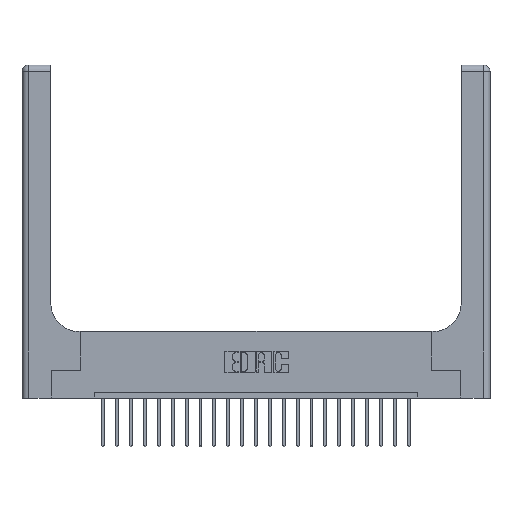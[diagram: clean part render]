
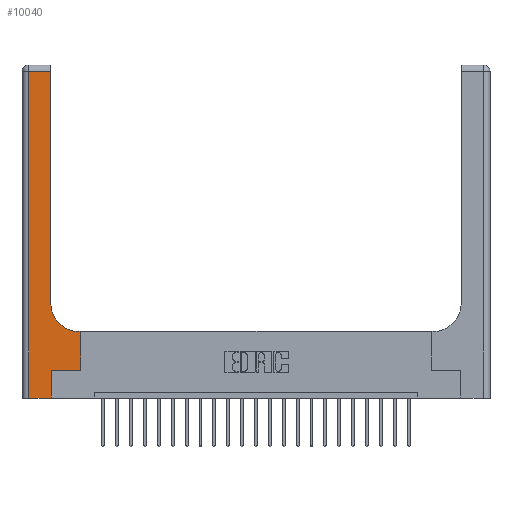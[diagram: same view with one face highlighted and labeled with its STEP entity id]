
A CAD part, top view. The second image highlights one B-rep face of the part: STEP entity #10040.
In plain terms, the highlighted planar face has unit normal (0, 0, 1).
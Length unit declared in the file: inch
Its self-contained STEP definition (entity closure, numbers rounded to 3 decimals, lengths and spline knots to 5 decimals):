
#422 = EDGE_CURVE ( 'NONE', #13824, #6355, #600, .T. ) ;
#600 = LINE ( 'NONE', #7864, #15520 ) ;
#1306 = VECTOR ( 'NONE', #3879, 39.37008 ) ;
#1350 = ORIENTED_EDGE ( 'NONE', *, *, #422, .T. ) ;
#1509 = DIRECTION ( 'NONE',  ( -1., 0., 0. ) ) ;
#1542 = ORIENTED_EDGE ( 'NONE', *, *, #16143, .T. ) ;
#1742 = CARTESIAN_POINT ( 'NONE',  ( 0.528, 0.25, 0.37 ) ) ;
#1911 = ORIENTED_EDGE ( 'NONE', *, *, #18647, .T. ) ;
#3413 = CARTESIAN_POINT ( 'NONE',  ( 0.51, 0.6, 0.37 ) ) ;
#3441 = DIRECTION ( 'NONE',  ( 0., 1., 0. ) ) ;
#3488 = AXIS2_PLACEMENT_3D ( 'NONE', #11070, #20191, #18031 ) ;
#3821 = VECTOR ( 'NONE', #7078, 39.37008 ) ;
#3879 = DIRECTION ( 'NONE',  ( 0., 1., 0. ) ) ;
#4105 = CARTESIAN_POINT ( 'NONE',  ( 0.06, 0., 0.37 ) ) ;
#4559 = LINE ( 'NONE', #14775, #11260 ) ;
#4609 = LINE ( 'NONE', #16997, #16040 ) ;
#4688 = CARTESIAN_POINT ( 'NONE',  ( 0.528, 0.25, 0.37 ) ) ;
#5566 = PLANE ( 'NONE',  #7668 ) ;
#5663 = VECTOR ( 'NONE', #21361, 39.37008 ) ;
#6355 = VERTEX_POINT ( 'NONE', #4105 ) ;
#7029 = VERTEX_POINT ( 'NONE', #4688 ) ;
#7078 = DIRECTION ( 'NONE',  ( -1., 0., 0. ) ) ;
#7214 = EDGE_CURVE ( 'NONE', #20038, #16830, #14089, .T. ) ;
#7511 = CARTESIAN_POINT ( 'NONE',  ( 0.26, 0.85, 0.37 ) ) ;
#7668 = AXIS2_PLACEMENT_3D ( 'NONE', #15899, #13770, #1509 ) ;
#7864 = CARTESIAN_POINT ( 'NONE',  ( 0.06, 3., 0.37 ) ) ;
#8215 = EDGE_CURVE ( 'NONE', #7029, #13641, #22311, .T. ) ;
#8663 = VERTEX_POINT ( 'NONE', #3413 ) ;
#8960 = CARTESIAN_POINT ( 'NONE',  ( 0.265, 0.25, 0.37 ) ) ;
#9094 = LINE ( 'NONE', #17748, #21242 ) ;
#9888 = DIRECTION ( 'NONE',  ( -1., 0., 0. ) ) ;
#10040 = ADVANCED_FACE ( 'NONE', ( #21147 ), #5566, .F. ) ;
#10306 = ORIENTED_EDGE ( 'NONE', *, *, #10682, .T. ) ;
#10348 = CARTESIAN_POINT ( 'NONE',  ( 0.06, 2.94, 0.37 ) ) ;
#10359 = CARTESIAN_POINT ( 'NONE',  ( 0.26, 0.6, 0.37 ) ) ;
#10680 = CARTESIAN_POINT ( 'NONE',  ( 0.265, 0., 0.37 ) ) ;
#10682 = EDGE_CURVE ( 'NONE', #6355, #20038, #4609, .T. ) ;
#10888 = ORIENTED_EDGE ( 'NONE', *, *, #16831, .T. ) ;
#11070 = CARTESIAN_POINT ( 'NONE',  ( 0.51, 0.85, 0.37 ) ) ;
#11137 = EDGE_CURVE ( 'NONE', #14824, #13824, #4559, .T. ) ;
#11260 = VECTOR ( 'NONE', #9888, 39.37008 ) ;
#12115 = CARTESIAN_POINT ( 'NONE',  ( 0.528, 0.6, 0.37 ) ) ;
#12662 = ORIENTED_EDGE ( 'NONE', *, *, #11137, .T. ) ;
#12752 = DIRECTION ( 'NONE',  ( 0., -1., 0. ) ) ;
#13272 = CIRCLE ( 'NONE', #3488, 0.25 ) ;
#13641 = VERTEX_POINT ( 'NONE', #12115 ) ;
#13657 = LINE ( 'NONE', #10359, #3821 ) ;
#13687 = DIRECTION ( 'NONE',  ( 1., 0., 0. ) ) ;
#13770 = DIRECTION ( 'NONE',  ( 0., 0., -1. ) ) ;
#13824 = VERTEX_POINT ( 'NONE', #10348 ) ;
#13974 = VERTEX_POINT ( 'NONE', #7511 ) ;
#14089 = LINE ( 'NONE', #10680, #1306 ) ;
#14172 = LINE ( 'NONE', #15785, #5663 ) ;
#14683 = EDGE_LOOP ( 'NONE', ( #10888, #12662, #1350, #10306, #16465, #15661, #21890, #1542, #1911 ) ) ;
#14775 = CARTESIAN_POINT ( 'NONE',  ( 0., 2.94, 0.37 ) ) ;
#14824 = VERTEX_POINT ( 'NONE', #21982 ) ;
#15520 = VECTOR ( 'NONE', #12752, 39.37008 ) ;
#15661 = ORIENTED_EDGE ( 'NONE', *, *, #17598, .T. ) ;
#15785 = CARTESIAN_POINT ( 'NONE',  ( 0.26, 3., 0.37 ) ) ;
#15899 = CARTESIAN_POINT ( 'NONE',  ( 0., 3., 0.37 ) ) ;
#16040 = VECTOR ( 'NONE', #13687, 39.37008 ) ;
#16143 = EDGE_CURVE ( 'NONE', #13641, #8663, #13657, .T. ) ;
#16465 = ORIENTED_EDGE ( 'NONE', *, *, #7214, .T. ) ;
#16830 = VERTEX_POINT ( 'NONE', #8960 ) ;
#16831 = EDGE_CURVE ( 'NONE', #13974, #14824, #14172, .T. ) ;
#16997 = CARTESIAN_POINT ( 'NONE',  ( 0., 0., 0.37 ) ) ;
#17598 = EDGE_CURVE ( 'NONE', #16830, #7029, #9094, .T. ) ;
#17748 = CARTESIAN_POINT ( 'NONE',  ( 0.265, 0.25, 0.37 ) ) ;
#17934 = VECTOR ( 'NONE', #3441, 39.37008 ) ;
#18031 = DIRECTION ( 'NONE',  ( 1., 0., 0. ) ) ;
#18647 = EDGE_CURVE ( 'NONE', #8663, #13974, #13272, .T. ) ;
#20038 = VERTEX_POINT ( 'NONE', #22431 ) ;
#20191 = DIRECTION ( 'NONE',  ( 0., 0., -1. ) ) ;
#21147 = FACE_OUTER_BOUND ( 'NONE', #14683, .T. ) ;
#21175 = DIRECTION ( 'NONE',  ( 1., 0., 0. ) ) ;
#21242 = VECTOR ( 'NONE', #21175, 39.37008 ) ;
#21361 = DIRECTION ( 'NONE',  ( 0., 1., 0. ) ) ;
#21890 = ORIENTED_EDGE ( 'NONE', *, *, #8215, .T. ) ;
#21982 = CARTESIAN_POINT ( 'NONE',  ( 0.26, 2.94, 0.37 ) ) ;
#22311 = LINE ( 'NONE', #1742, #17934 ) ;
#22431 = CARTESIAN_POINT ( 'NONE',  ( 0.265, 0., 0.37 ) ) ;
